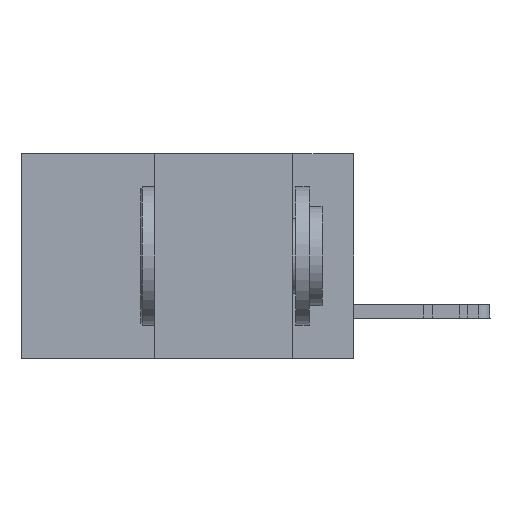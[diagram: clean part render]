
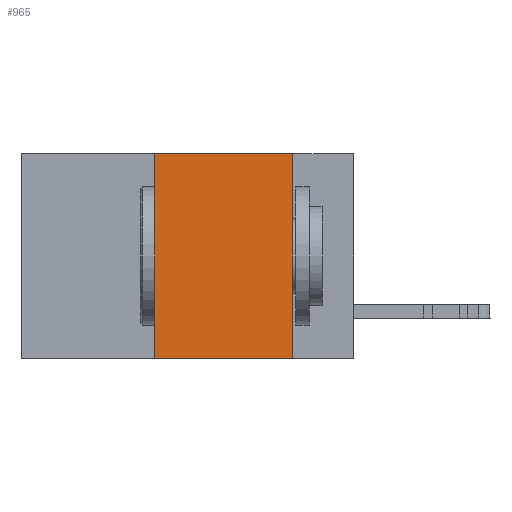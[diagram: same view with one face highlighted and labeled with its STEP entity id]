
A CAD part, left-side view. The second image highlights one B-rep face of the part: STEP entity #965.
In plain terms, the highlighted planar face has unit normal (-1, 0, 0).
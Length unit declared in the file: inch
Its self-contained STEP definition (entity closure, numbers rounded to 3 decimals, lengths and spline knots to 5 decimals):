
#965 = ADVANCED_FACE ( 'NONE', ( #11887 ), #41011, .F. ) ;
#1232 = VECTOR ( 'NONE', #12742, 39.37008 ) ;
#2735 = AXIS2_PLACEMENT_3D ( 'NONE', #16342, #31449, #21443 ) ;
#3381 = DIRECTION ( 'NONE',  ( 0., -1., 0. ) ) ;
#3497 = EDGE_CURVE ( 'NONE', #42308, #22376, #29264, .T. ) ;
#6318 = DIRECTION ( 'NONE',  ( 0., 0., -1. ) ) ;
#7041 = VERTEX_POINT ( 'NONE', #33036 ) ;
#7229 = ORIENTED_EDGE ( 'NONE', *, *, #3497, .F. ) ;
#8746 = ORIENTED_EDGE ( 'NONE', *, *, #23573, .F. ) ;
#9450 = ORIENTED_EDGE ( 'NONE', *, *, #11805, .T. ) ;
#10140 = EDGE_LOOP ( 'NONE', ( #7229, #32885, #8746, #9450 ) ) ;
#10527 = LINE ( 'NONE', #21087, #31543 ) ;
#11805 = EDGE_CURVE ( 'NONE', #7041, #22376, #10527, .T. ) ;
#11887 = FACE_OUTER_BOUND ( 'NONE', #10140, .T. ) ;
#12509 = VERTEX_POINT ( 'NONE', #24663 ) ;
#12742 = DIRECTION ( 'NONE',  ( 0., -1., 0. ) ) ;
#16342 = CARTESIAN_POINT ( 'NONE',  ( 0., 0.6, 0. ) ) ;
#16807 = CARTESIAN_POINT ( 'NONE',  ( 0., 0.11, 0. ) ) ;
#16852 = VECTOR ( 'NONE', #6318, 39.37008 ) ;
#17099 = EDGE_CURVE ( 'NONE', #12509, #42308, #22362, .T. ) ;
#21087 = CARTESIAN_POINT ( 'NONE',  ( 0., 0.6, -0.37 ) ) ;
#21443 = DIRECTION ( 'NONE',  ( 0., 0., -1. ) ) ;
#22362 = LINE ( 'NONE', #24232, #1232 ) ;
#22376 = VERTEX_POINT ( 'NONE', #36154 ) ;
#23573 = EDGE_CURVE ( 'NONE', #7041, #12509, #41927, .T. ) ;
#24232 = CARTESIAN_POINT ( 'NONE',  ( 0., 0.6, 0. ) ) ;
#24663 = CARTESIAN_POINT ( 'NONE',  ( 0., 0.36, 0. ) ) ;
#26798 = CARTESIAN_POINT ( 'NONE',  ( 0., 0.11, 0. ) ) ;
#29264 = LINE ( 'NONE', #16807, #16852 ) ;
#31449 = DIRECTION ( 'NONE',  ( 1., 0., 0. ) ) ;
#31543 = VECTOR ( 'NONE', #3381, 39.37008 ) ;
#31709 = CARTESIAN_POINT ( 'NONE',  ( 0., 0.36, 0. ) ) ;
#32885 = ORIENTED_EDGE ( 'NONE', *, *, #17099, .F. ) ;
#33036 = CARTESIAN_POINT ( 'NONE',  ( 0., 0.36, -0.37 ) ) ;
#35311 = DIRECTION ( 'NONE',  ( 0., 0., 1. ) ) ;
#36154 = CARTESIAN_POINT ( 'NONE',  ( 0., 0.11, -0.37 ) ) ;
#41011 = PLANE ( 'NONE',  #2735 ) ;
#41927 = LINE ( 'NONE', #31709, #45460 ) ;
#42308 = VERTEX_POINT ( 'NONE', #26798 ) ;
#45460 = VECTOR ( 'NONE', #35311, 39.37008 ) ;
